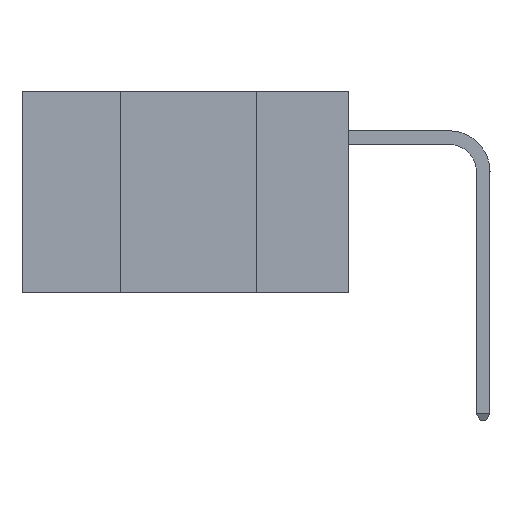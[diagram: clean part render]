
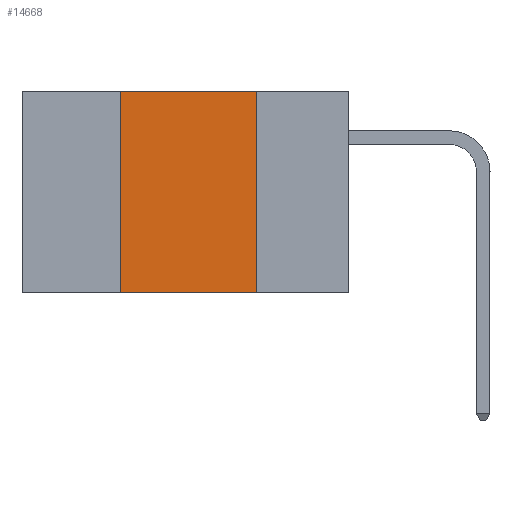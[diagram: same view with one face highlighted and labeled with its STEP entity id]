
A CAD part, left-side view. The second image highlights one B-rep face of the part: STEP entity #14668.
In plain terms, the highlighted planar face has unit normal (-1, 0, 0).
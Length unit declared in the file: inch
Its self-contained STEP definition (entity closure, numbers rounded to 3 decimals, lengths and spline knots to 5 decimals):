
#338 = VECTOR ( 'NONE', #9379, 39.37008 ) ;
#351 = CARTESIAN_POINT ( 'NONE',  ( 0., 0.42, 0. ) ) ;
#1174 = LINE ( 'NONE', #40985, #39317 ) ;
#2445 = ORIENTED_EDGE ( 'NONE', *, *, #46616, .F. ) ;
#2578 = EDGE_LOOP ( 'NONE', ( #27649, #2445, #5926, #7712 ) ) ;
#5926 = ORIENTED_EDGE ( 'NONE', *, *, #28375, .F. ) ;
#7712 = ORIENTED_EDGE ( 'NONE', *, *, #46530, .T. ) ;
#7817 = PLANE ( 'NONE',  #29414 ) ;
#9379 = DIRECTION ( 'NONE',  ( 0., -1., 0. ) ) ;
#10503 = CARTESIAN_POINT ( 'NONE',  ( 0., 0.17, -0.37 ) ) ;
#11485 = DIRECTION ( 'NONE',  ( 0., 0., -1. ) ) ;
#11550 = DIRECTION ( 'NONE',  ( 1., 0., 0. ) ) ;
#13591 = DIRECTION ( 'NONE',  ( 0., -1., 0. ) ) ;
#14668 = ADVANCED_FACE ( 'NONE', ( #40439 ), #7817, .F. ) ;
#15531 = DIRECTION ( 'NONE',  ( 0., 0., 1. ) ) ;
#16052 = EDGE_CURVE ( 'NONE', #40651, #31105, #1174, .T. ) ;
#20093 = LINE ( 'NONE', #20406, #338 ) ;
#20406 = CARTESIAN_POINT ( 'NONE',  ( 0., 0.6, -0.37 ) ) ;
#20602 = VECTOR ( 'NONE', #15531, 39.37008 ) ;
#25234 = VECTOR ( 'NONE', #13591, 39.37008 ) ;
#27649 = ORIENTED_EDGE ( 'NONE', *, *, #16052, .F. ) ;
#28129 = CARTESIAN_POINT ( 'NONE',  ( 0., 0.6, 0. ) ) ;
#28375 = EDGE_CURVE ( 'NONE', #40731, #36536, #39006, .T. ) ;
#29414 = AXIS2_PLACEMENT_3D ( 'NONE', #33643, #11550, #37306 ) ;
#31105 = VERTEX_POINT ( 'NONE', #10503 ) ;
#33643 = CARTESIAN_POINT ( 'NONE',  ( 0., 0.6, 0. ) ) ;
#35002 = LINE ( 'NONE', #28129, #25234 ) ;
#36536 = VERTEX_POINT ( 'NONE', #351 ) ;
#37306 = DIRECTION ( 'NONE',  ( 0., 0., -1. ) ) ;
#37526 = CARTESIAN_POINT ( 'NONE',  ( 0., 0.42, 0. ) ) ;
#39006 = LINE ( 'NONE', #37526, #20602 ) ;
#39317 = VECTOR ( 'NONE', #11485, 39.37008 ) ;
#40133 = CARTESIAN_POINT ( 'NONE',  ( 0., 0.17, 0. ) ) ;
#40439 = FACE_OUTER_BOUND ( 'NONE', #2578, .T. ) ;
#40604 = CARTESIAN_POINT ( 'NONE',  ( 0., 0.42, -0.37 ) ) ;
#40651 = VERTEX_POINT ( 'NONE', #40133 ) ;
#40731 = VERTEX_POINT ( 'NONE', #40604 ) ;
#40985 = CARTESIAN_POINT ( 'NONE',  ( 0., 0.17, 0. ) ) ;
#46530 = EDGE_CURVE ( 'NONE', #40731, #31105, #20093, .T. ) ;
#46616 = EDGE_CURVE ( 'NONE', #36536, #40651, #35002, .T. ) ;
